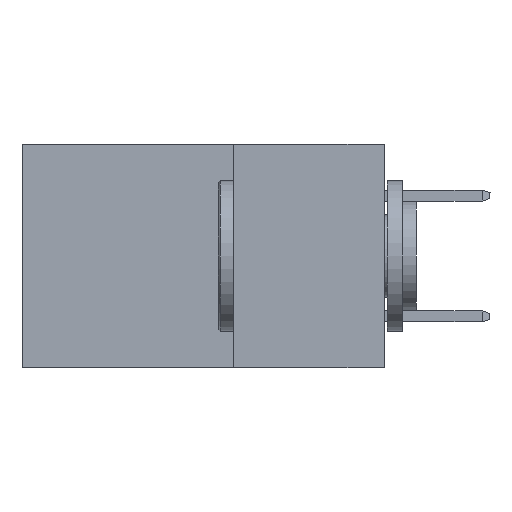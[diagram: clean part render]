
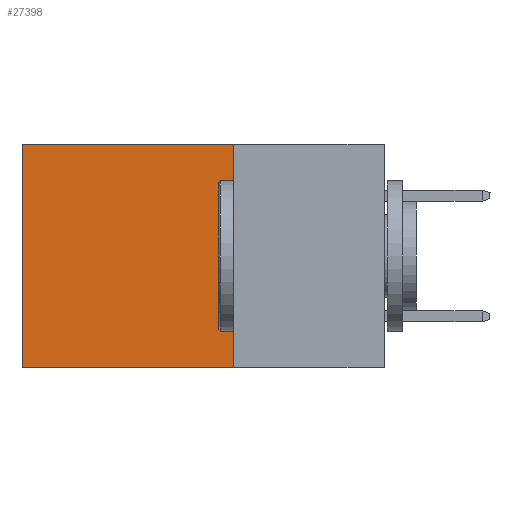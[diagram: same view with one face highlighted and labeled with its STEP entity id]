
A CAD part, left-side view. The second image highlights one B-rep face of the part: STEP entity #27398.
In plain terms, the highlighted planar face has unit normal (-1, 0, 0).
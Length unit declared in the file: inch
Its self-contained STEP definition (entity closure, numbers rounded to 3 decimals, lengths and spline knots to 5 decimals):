
#464 = CARTESIAN_POINT ( 'NONE',  ( 0.298, 0.6, -0.37 ) ) ;
#1264 = ORIENTED_EDGE ( 'NONE', *, *, #24848, .F. ) ;
#2697 = EDGE_CURVE ( 'NONE', #20618, #21279, #14700, .T. ) ;
#3281 = DIRECTION ( 'NONE',  ( 1., 0., 0. ) ) ;
#3645 = FACE_OUTER_BOUND ( 'NONE', #21429, .T. ) ;
#3676 = VERTEX_POINT ( 'NONE', #19328 ) ;
#4134 = CARTESIAN_POINT ( 'NONE',  ( 0.298, 0.6, 0. ) ) ;
#4605 = CARTESIAN_POINT ( 'NONE',  ( 0.298, 0.25, 0. ) ) ;
#4894 = ORIENTED_EDGE ( 'NONE', *, *, #2697, .F. ) ;
#7273 = LINE ( 'NONE', #4134, #19833 ) ;
#7582 = EDGE_CURVE ( 'NONE', #14154, #21279, #7273, .T. ) ;
#7724 = LINE ( 'NONE', #4605, #24937 ) ;
#9692 = CARTESIAN_POINT ( 'NONE',  ( 0.298, 0.25, 0. ) ) ;
#11896 = CARTESIAN_POINT ( 'NONE',  ( 0.298, 0.25, 0. ) ) ;
#12550 = DIRECTION ( 'NONE',  ( 0., 0., -1. ) ) ;
#13872 = VECTOR ( 'NONE', #16253, 39.37008 ) ;
#13919 = DIRECTION ( 'NONE',  ( 0., 0., -1. ) ) ;
#14154 = VERTEX_POINT ( 'NONE', #17580 ) ;
#14700 = LINE ( 'NONE', #27109, #23348 ) ;
#16253 = DIRECTION ( 'NONE',  ( 0., 1., 0. ) ) ;
#17580 = CARTESIAN_POINT ( 'NONE',  ( 0.298, 0.6, 0. ) ) ;
#18647 = DIRECTION ( 'NONE',  ( 0., 1., 0. ) ) ;
#19137 = ORIENTED_EDGE ( 'NONE', *, *, #20593, .T. ) ;
#19328 = CARTESIAN_POINT ( 'NONE',  ( 0.298, 0.25, 0. ) ) ;
#19833 = VECTOR ( 'NONE', #12550, 39.37008 ) ;
#20252 = PLANE ( 'NONE',  #24360 ) ;
#20351 = CARTESIAN_POINT ( 'NONE',  ( 0.298, 0.25, -0.37 ) ) ;
#20593 = EDGE_CURVE ( 'NONE', #3676, #14154, #21851, .T. ) ;
#20618 = VERTEX_POINT ( 'NONE', #20351 ) ;
#21279 = VERTEX_POINT ( 'NONE', #464 ) ;
#21429 = EDGE_LOOP ( 'NONE', ( #25472, #4894, #1264, #19137 ) ) ;
#21851 = LINE ( 'NONE', #9692, #13872 ) ;
#23348 = VECTOR ( 'NONE', #18647, 39.37008 ) ;
#23681 = DIRECTION ( 'NONE',  ( 0., 0., -1. ) ) ;
#24360 = AXIS2_PLACEMENT_3D ( 'NONE', #11896, #3281, #13919 ) ;
#24848 = EDGE_CURVE ( 'NONE', #3676, #20618, #7724, .T. ) ;
#24937 = VECTOR ( 'NONE', #23681, 39.37008 ) ;
#25472 = ORIENTED_EDGE ( 'NONE', *, *, #7582, .T. ) ;
#27109 = CARTESIAN_POINT ( 'NONE',  ( 0.298, 0.25, -0.37 ) ) ;
#27398 = ADVANCED_FACE ( 'NONE', ( #3645 ), #20252, .F. ) ;
